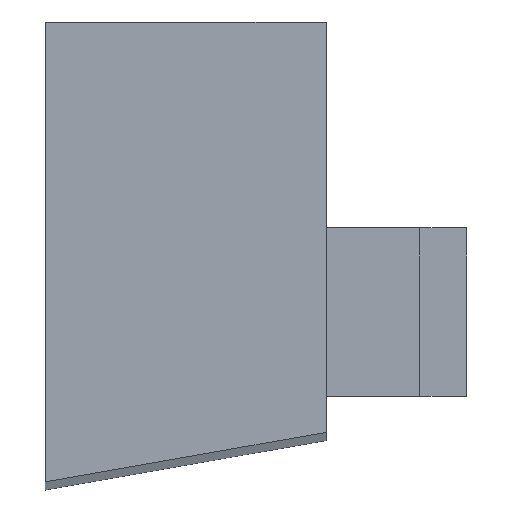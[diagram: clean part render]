
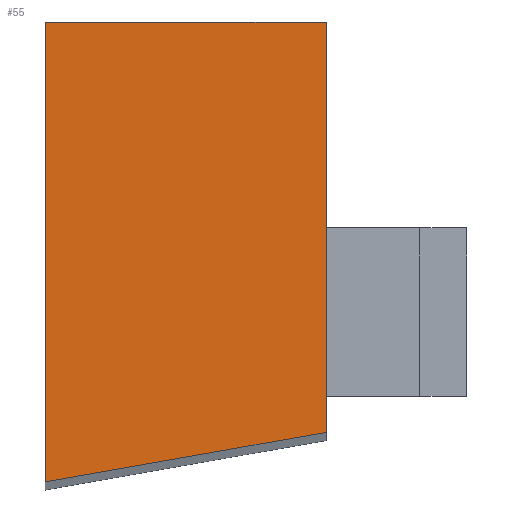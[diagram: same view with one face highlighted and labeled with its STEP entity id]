
A CAD part, left-side view. The second image highlights one B-rep face of the part: STEP entity #55.
In plain terms, the highlighted planar face has unit normal (-1, 0, 0).
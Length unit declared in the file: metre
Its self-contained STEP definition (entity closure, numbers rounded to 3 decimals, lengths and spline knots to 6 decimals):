
#55 = ADVANCED_FACE( '', ( #111 ), #112, .F. );
#111 = FACE_OUTER_BOUND( '', #164, .T. );
#112 = PLANE( '', #165 );
#164 = EDGE_LOOP( '', ( #258, #259, #260, #261 ) );
#165 = AXIS2_PLACEMENT_3D( '', #262, #263, #264 );
#258 = ORIENTED_EDGE( '', *, *, #346, .T. );
#259 = ORIENTED_EDGE( '', *, *, #357, .F. );
#260 = ORIENTED_EDGE( '', *, *, #331, .F. );
#261 = ORIENTED_EDGE( '', *, *, #358, .T. );
#262 = CARTESIAN_POINT( '', ( 0., 0.00762, -0.012478 ) );
#263 = DIRECTION( '', ( 1., 0., 0. ) );
#264 = DIRECTION( '', ( 0., 0., -1. ) );
#331 = EDGE_CURVE( '', #392, #393, #394, .T. );
#346 = EDGE_CURVE( '', #413, #417, #419, .T. );
#357 = EDGE_CURVE( '', #393, #417, #432, .T. );
#358 = EDGE_CURVE( '', #392, #413, #433, .F. );
#392 = VERTEX_POINT( '', #478 );
#393 = VERTEX_POINT( '', #479 );
#394 = LINE( '', #480, #481 );
#413 = VERTEX_POINT( '', #509 );
#417 = VERTEX_POINT( '', #515 );
#419 = LINE( '', #518, #519 );
#432 = LINE( '', #538, #539 );
#433 = LINE( '', #540, #541 );
#478 = CARTESIAN_POINT( '', ( 0., 0.00762, -0.012478 ) );
#479 = CARTESIAN_POINT( '', ( 0., 0.00762, 0. ) );
#480 = CARTESIAN_POINT( '', ( 0., 0.00762, -0.012478 ) );
#481 = VECTOR( '', #565, 1. );
#509 = CARTESIAN_POINT( '', ( 0., 0., -0.011135 ) );
#515 = CARTESIAN_POINT( '', ( 0., 0., 0. ) );
#518 = CARTESIAN_POINT( '', ( 0., 0., -0.012478 ) );
#519 = VECTOR( '', #578, 1. );
#538 = CARTESIAN_POINT( '', ( 0., 0.00762, 0. ) );
#539 = VECTOR( '', #585, 1. );
#540 = CARTESIAN_POINT( '', ( 0., 0.00762, -0.012478 ) );
#541 = VECTOR( '', #586, 1. );
#565 = DIRECTION( '', ( 0., 0., 1. ) );
#578 = DIRECTION( '', ( 0., 0., 1. ) );
#585 = DIRECTION( '', ( 0., -1., 0. ) );
#586 = DIRECTION( '', ( 0., 0.985, -0.174 ) );
